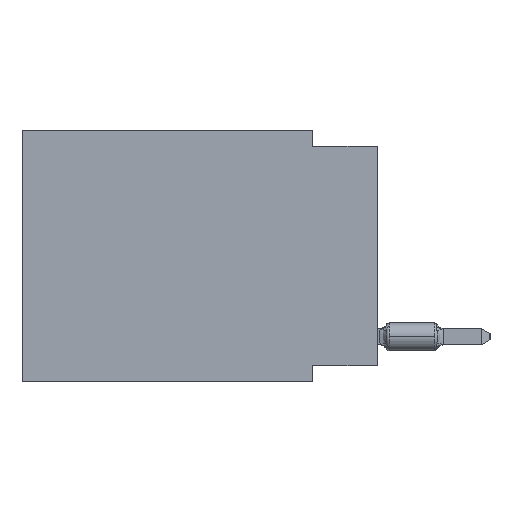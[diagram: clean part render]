
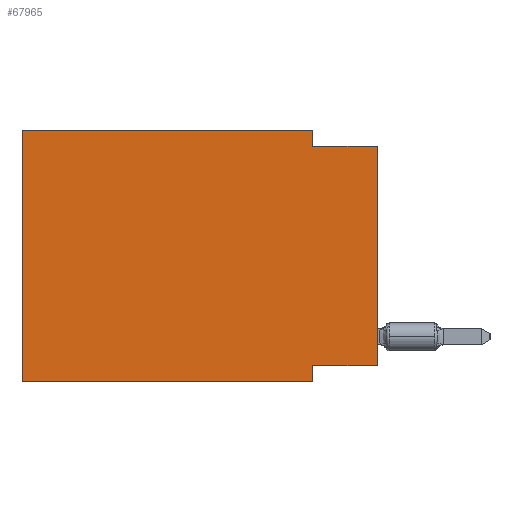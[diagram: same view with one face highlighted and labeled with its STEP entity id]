
A CAD part, left-side view. The second image highlights one B-rep face of the part: STEP entity #67965.
In plain terms, the highlighted planar face has unit normal (-1, 0, 0).
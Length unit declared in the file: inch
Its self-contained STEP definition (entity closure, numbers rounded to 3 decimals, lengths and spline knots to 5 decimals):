
#1753 = VECTOR ( 'NONE', #55852, 39.37008 ) ;
#1931 = DIRECTION ( 'NONE',  ( 0., 1., 0. ) ) ;
#2846 = DIRECTION ( 'NONE',  ( 0., -1., 0. ) ) ;
#6051 = VERTEX_POINT ( 'NONE', #28098 ) ;
#6212 = CARTESIAN_POINT ( 'NONE',  ( 0., 0.1, 0. ) ) ;
#6804 = EDGE_CURVE ( 'NONE', #22322, #74771, #25519, .T. ) ;
#7112 = ORIENTED_EDGE ( 'NONE', *, *, #43839, .T. ) ;
#8592 = CARTESIAN_POINT ( 'NONE',  ( 0., 0.55, 0. ) ) ;
#9783 = DIRECTION ( 'NONE',  ( 0., 0., -1. ) ) ;
#11872 = DIRECTION ( 'NONE',  ( 0., 0., -1. ) ) ;
#14544 = VECTOR ( 'NONE', #23906, 39.37008 ) ;
#14655 = ORIENTED_EDGE ( 'NONE', *, *, #47855, .F. ) ;
#16365 = EDGE_CURVE ( 'NONE', #40974, #74771, #22910, .T. ) ;
#17939 = DIRECTION ( 'NONE',  ( 0., -1., 0. ) ) ;
#18259 = CARTESIAN_POINT ( 'NONE',  ( 0., 0.55, -0.39 ) ) ;
#18359 = ORIENTED_EDGE ( 'NONE', *, *, #16365, .F. ) ;
#18519 = EDGE_LOOP ( 'NONE', ( #7112, #24799, #61263, #44380, #20743, #18978, #18359, #14655 ) ) ;
#18978 = ORIENTED_EDGE ( 'NONE', *, *, #6804, .T. ) ;
#20743 = ORIENTED_EDGE ( 'NONE', *, *, #45554, .F. ) ;
#22322 = VERTEX_POINT ( 'NONE', #39542 ) ;
#22431 = VERTEX_POINT ( 'NONE', #41141 ) ;
#22910 = LINE ( 'NONE', #35792, #29046 ) ;
#23609 = LINE ( 'NONE', #6212, #59574 ) ;
#23906 = DIRECTION ( 'NONE',  ( 0., 0., 1. ) ) ;
#24799 = ORIENTED_EDGE ( 'NONE', *, *, #70760, .F. ) ;
#25519 = LINE ( 'NONE', #18259, #1753 ) ;
#26759 = DIRECTION ( 'NONE',  ( 1., 0., 0. ) ) ;
#27558 = PLANE ( 'NONE',  #68326 ) ;
#27880 = CARTESIAN_POINT ( 'NONE',  ( 0., 0., -0.025 ) ) ;
#28098 = CARTESIAN_POINT ( 'NONE',  ( 0., 0., -0.025 ) ) ;
#29046 = VECTOR ( 'NONE', #42678, 39.37008 ) ;
#30021 = CARTESIAN_POINT ( 'NONE',  ( 0., 0.1, -0.365 ) ) ;
#31248 = VERTEX_POINT ( 'NONE', #76785 ) ;
#31429 = LINE ( 'NONE', #75875, #62657 ) ;
#35792 = CARTESIAN_POINT ( 'NONE',  ( 0., 0.1, -0.39 ) ) ;
#39542 = CARTESIAN_POINT ( 'NONE',  ( 0., 0.55, -0.39 ) ) ;
#39705 = FACE_OUTER_BOUND ( 'NONE', #18519, .T. ) ;
#40974 = VERTEX_POINT ( 'NONE', #30021 ) ;
#41141 = CARTESIAN_POINT ( 'NONE',  ( 0., 0.1, -0.025 ) ) ;
#42678 = DIRECTION ( 'NONE',  ( 0., 0., -1. ) ) ;
#42917 = VERTEX_POINT ( 'NONE', #77177 ) ;
#43839 = EDGE_CURVE ( 'NONE', #78832, #6051, #78487, .T. ) ;
#44380 = ORIENTED_EDGE ( 'NONE', *, *, #70633, .F. ) ;
#45554 = EDGE_CURVE ( 'NONE', #22322, #31248, #57170, .T. ) ;
#46720 = CARTESIAN_POINT ( 'NONE',  ( 0., 0.1, -0.39 ) ) ;
#46990 = VECTOR ( 'NONE', #69681, 39.37008 ) ;
#47855 = EDGE_CURVE ( 'NONE', #78832, #40974, #31429, .T. ) ;
#48257 = CARTESIAN_POINT ( 'NONE',  ( 0., 0.55, 0. ) ) ;
#49457 = LINE ( 'NONE', #48257, #63626 ) ;
#50257 = LINE ( 'NONE', #27880, #54632 ) ;
#51496 = CARTESIAN_POINT ( 'NONE',  ( 0., 0.55, 0. ) ) ;
#53848 = CARTESIAN_POINT ( 'NONE',  ( 0., 0., 0. ) ) ;
#54632 = VECTOR ( 'NONE', #2846, 39.37008 ) ;
#54689 = EDGE_CURVE ( 'NONE', #42917, #22431, #23609, .T. ) ;
#55852 = DIRECTION ( 'NONE',  ( 0., -1., 0. ) ) ;
#57170 = LINE ( 'NONE', #51496, #46990 ) ;
#59574 = VECTOR ( 'NONE', #11872, 39.37008 ) ;
#61263 = ORIENTED_EDGE ( 'NONE', *, *, #54689, .F. ) ;
#62657 = VECTOR ( 'NONE', #1931, 39.37008 ) ;
#63626 = VECTOR ( 'NONE', #17939, 39.37008 ) ;
#67965 = ADVANCED_FACE ( 'NONE', ( #39705 ), #27558, .F. ) ;
#68326 = AXIS2_PLACEMENT_3D ( 'NONE', #8592, #26759, #9783 ) ;
#69681 = DIRECTION ( 'NONE',  ( 0., 0., 1. ) ) ;
#70633 = EDGE_CURVE ( 'NONE', #31248, #42917, #49457, .T. ) ;
#70760 = EDGE_CURVE ( 'NONE', #22431, #6051, #50257, .T. ) ;
#74771 = VERTEX_POINT ( 'NONE', #46720 ) ;
#75875 = CARTESIAN_POINT ( 'NONE',  ( 0., 0., -0.365 ) ) ;
#76667 = CARTESIAN_POINT ( 'NONE',  ( 0., 0., -0.365 ) ) ;
#76785 = CARTESIAN_POINT ( 'NONE',  ( 0., 0.55, 0. ) ) ;
#77177 = CARTESIAN_POINT ( 'NONE',  ( 0., 0.1, 0. ) ) ;
#78487 = LINE ( 'NONE', #53848, #14544 ) ;
#78832 = VERTEX_POINT ( 'NONE', #76667 ) ;
